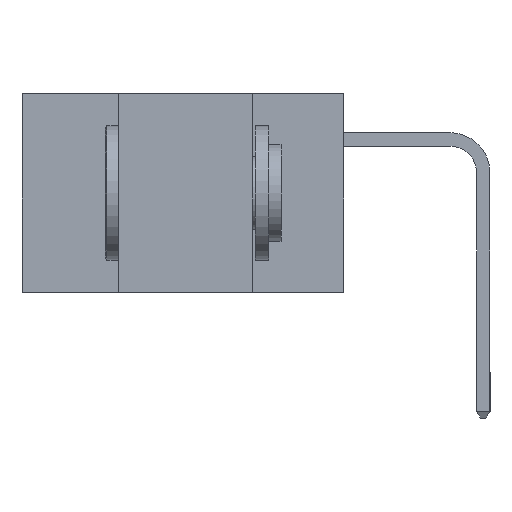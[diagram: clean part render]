
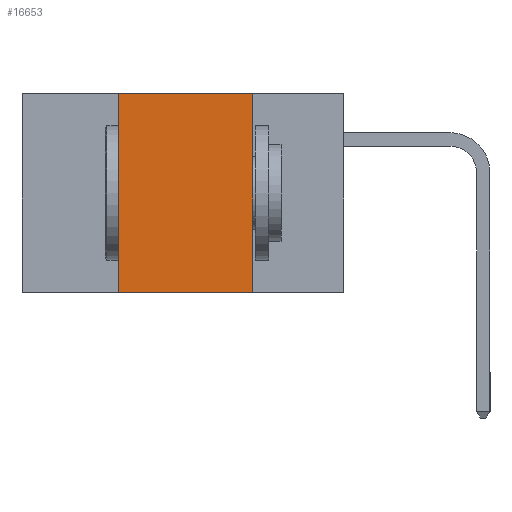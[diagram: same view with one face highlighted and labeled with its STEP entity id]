
A CAD part, left-side view. The second image highlights one B-rep face of the part: STEP entity #16653.
In plain terms, the highlighted planar face has unit normal (-1, 0, 0).
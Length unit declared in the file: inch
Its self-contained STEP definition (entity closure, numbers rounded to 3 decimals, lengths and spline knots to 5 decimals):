
#1050 = PLANE ( 'NONE',  #12354 ) ;
#1692 = ORIENTED_EDGE ( 'NONE', *, *, #14879, .F. ) ;
#1885 = VECTOR ( 'NONE', #11113, 39.37008 ) ;
#2009 = ORIENTED_EDGE ( 'NONE', *, *, #20237, .F. ) ;
#2385 = CARTESIAN_POINT ( 'NONE',  ( 0., 0.17, 0. ) ) ;
#2725 = EDGE_LOOP ( 'NONE', ( #2009, #1692, #15721, #2978 ) ) ;
#2900 = LINE ( 'NONE', #9588, #1885 ) ;
#2978 = ORIENTED_EDGE ( 'NONE', *, *, #17612, .T. ) ;
#3668 = CARTESIAN_POINT ( 'NONE',  ( 0., 0.42, 0. ) ) ;
#4458 = LINE ( 'NONE', #9602, #19365 ) ;
#5323 = VERTEX_POINT ( 'NONE', #3668 ) ;
#7746 = CARTESIAN_POINT ( 'NONE',  ( 0., 0.6, 0. ) ) ;
#9588 = CARTESIAN_POINT ( 'NONE',  ( 0., 0.17, -0.37 ) ) ;
#9602 = CARTESIAN_POINT ( 'NONE',  ( 0., 0.6, 0. ) ) ;
#9998 = LINE ( 'NONE', #12959, #16618 ) ;
#10596 = CARTESIAN_POINT ( 'NONE',  ( 0., 0.42, -0.37 ) ) ;
#10635 = EDGE_CURVE ( 'NONE', #19537, #5323, #20999, .T. ) ;
#11027 = DIRECTION ( 'NONE',  ( 0., -1., 0. ) ) ;
#11113 = DIRECTION ( 'NONE',  ( 0., 0., -1. ) ) ;
#12354 = AXIS2_PLACEMENT_3D ( 'NONE', #7746, #14439, #14552 ) ;
#12934 = CARTESIAN_POINT ( 'NONE',  ( 0., 0.42, -0.37 ) ) ;
#12959 = CARTESIAN_POINT ( 'NONE',  ( 0., 0.6, -0.37 ) ) ;
#13138 = VECTOR ( 'NONE', #16038, 39.37008 ) ;
#14439 = DIRECTION ( 'NONE',  ( 1., 0., 0. ) ) ;
#14552 = DIRECTION ( 'NONE',  ( 0., 0., -1. ) ) ;
#14715 = DIRECTION ( 'NONE',  ( 0., -1., 0. ) ) ;
#14879 = EDGE_CURVE ( 'NONE', #5323, #19654, #4458, .T. ) ;
#15237 = VERTEX_POINT ( 'NONE', #20941 ) ;
#15721 = ORIENTED_EDGE ( 'NONE', *, *, #10635, .F. ) ;
#16038 = DIRECTION ( 'NONE',  ( 0., 0., 1. ) ) ;
#16101 = FACE_OUTER_BOUND ( 'NONE', #2725, .T. ) ;
#16618 = VECTOR ( 'NONE', #14715, 39.37008 ) ;
#16653 = ADVANCED_FACE ( 'NONE', ( #16101 ), #1050, .F. ) ;
#17612 = EDGE_CURVE ( 'NONE', #19537, #15237, #9998, .T. ) ;
#19365 = VECTOR ( 'NONE', #11027, 39.37008 ) ;
#19537 = VERTEX_POINT ( 'NONE', #10596 ) ;
#19654 = VERTEX_POINT ( 'NONE', #2385 ) ;
#20237 = EDGE_CURVE ( 'NONE', #19654, #15237, #2900, .T. ) ;
#20941 = CARTESIAN_POINT ( 'NONE',  ( 0., 0.17, -0.37 ) ) ;
#20999 = LINE ( 'NONE', #12934, #13138 ) ;
